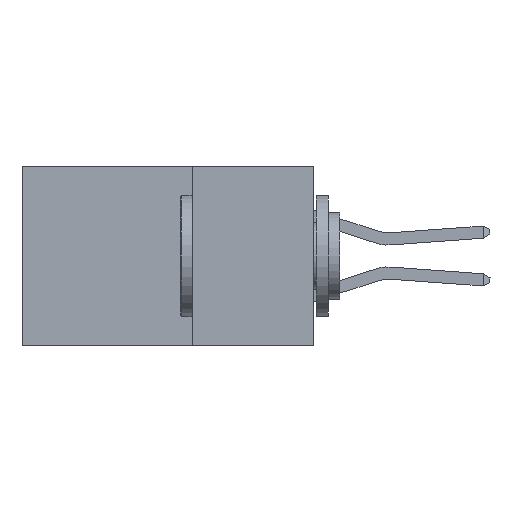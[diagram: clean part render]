
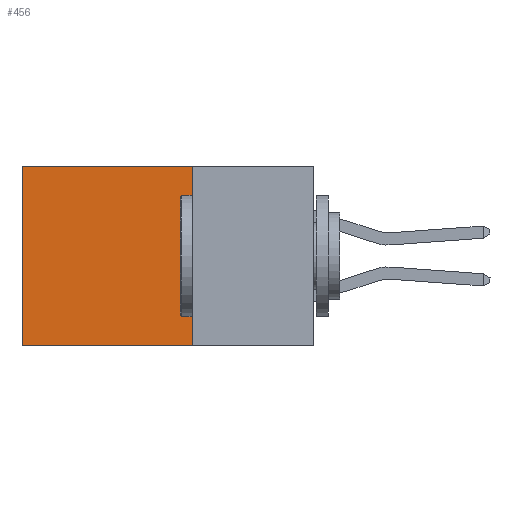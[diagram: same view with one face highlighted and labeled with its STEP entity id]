
A CAD part, left-side view. The second image highlights one B-rep face of the part: STEP entity #456.
In plain terms, the highlighted planar face has unit normal (-1, 0, 0).
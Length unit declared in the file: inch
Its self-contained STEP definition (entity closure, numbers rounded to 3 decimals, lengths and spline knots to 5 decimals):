
#38 = LINE ( 'NONE', #8024, #1478 ) ;
#456 = ADVANCED_FACE ( 'NONE', ( #12952 ), #13433, .F. ) ;
#1314 = VERTEX_POINT ( 'NONE', #5463 ) ;
#1478 = VECTOR ( 'NONE', #4703, 39.37008 ) ;
#1753 = CARTESIAN_POINT ( 'NONE',  ( 0.2875, 0.25, 0. ) ) ;
#1842 = VECTOR ( 'NONE', #7933, 39.37008 ) ;
#3070 = EDGE_LOOP ( 'NONE', ( #8213, #11944, #8025, #11834 ) ) ;
#3978 = CARTESIAN_POINT ( 'NONE',  ( 0.2875, 0.25, 0. ) ) ;
#4003 = DIRECTION ( 'NONE',  ( 0., 0., -1. ) ) ;
#4187 = VECTOR ( 'NONE', #13303, 39.37008 ) ;
#4703 = DIRECTION ( 'NONE',  ( 0., 1., 0. ) ) ;
#5463 = CARTESIAN_POINT ( 'NONE',  ( 0.2875, 0.25, -0.37 ) ) ;
#5669 = CARTESIAN_POINT ( 'NONE',  ( 0.2875, 0.6, -0.37 ) ) ;
#5753 = EDGE_CURVE ( 'NONE', #1314, #10822, #38, .T. ) ;
#5958 = CARTESIAN_POINT ( 'NONE',  ( 0.2875, 0.6, 0. ) ) ;
#5979 = LINE ( 'NONE', #1753, #1842 ) ;
#6270 = VERTEX_POINT ( 'NONE', #9016 ) ;
#6663 = LINE ( 'NONE', #3978, #4187 ) ;
#7164 = DIRECTION ( 'NONE',  ( 1., 0., 0. ) ) ;
#7933 = DIRECTION ( 'NONE',  ( 0., 1., 0. ) ) ;
#8024 = CARTESIAN_POINT ( 'NONE',  ( 0.2875, 0.25, -0.37 ) ) ;
#8025 = ORIENTED_EDGE ( 'NONE', *, *, #8692, .F. ) ;
#8213 = ORIENTED_EDGE ( 'NONE', *, *, #10444, .T. ) ;
#8268 = DIRECTION ( 'NONE',  ( 0., 0., -1. ) ) ;
#8692 = EDGE_CURVE ( 'NONE', #6270, #1314, #6663, .T. ) ;
#9016 = CARTESIAN_POINT ( 'NONE',  ( 0.2875, 0.25, 0. ) ) ;
#9206 = AXIS2_PLACEMENT_3D ( 'NONE', #9256, #7164, #8268 ) ;
#9256 = CARTESIAN_POINT ( 'NONE',  ( 0.2875, 0.25, 0. ) ) ;
#10444 = EDGE_CURVE ( 'NONE', #11926, #10822, #10579, .T. ) ;
#10579 = LINE ( 'NONE', #5958, #11231 ) ;
#10800 = CARTESIAN_POINT ( 'NONE',  ( 0.2875, 0.6, 0. ) ) ;
#10822 = VERTEX_POINT ( 'NONE', #5669 ) ;
#11231 = VECTOR ( 'NONE', #4003, 39.37008 ) ;
#11701 = EDGE_CURVE ( 'NONE', #6270, #11926, #5979, .T. ) ;
#11834 = ORIENTED_EDGE ( 'NONE', *, *, #11701, .T. ) ;
#11926 = VERTEX_POINT ( 'NONE', #10800 ) ;
#11944 = ORIENTED_EDGE ( 'NONE', *, *, #5753, .F. ) ;
#12952 = FACE_OUTER_BOUND ( 'NONE', #3070, .T. ) ;
#13303 = DIRECTION ( 'NONE',  ( 0., 0., -1. ) ) ;
#13433 = PLANE ( 'NONE',  #9206 ) ;
